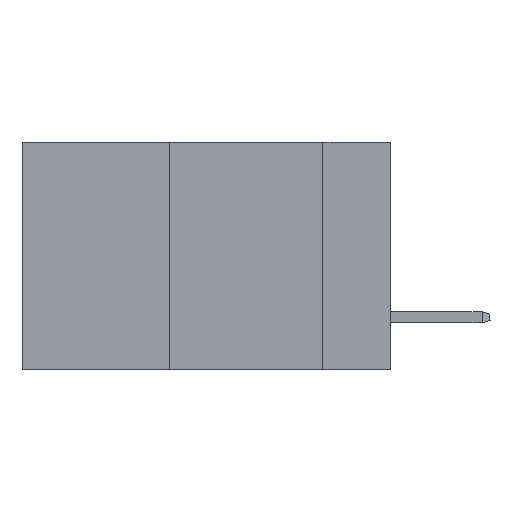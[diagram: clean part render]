
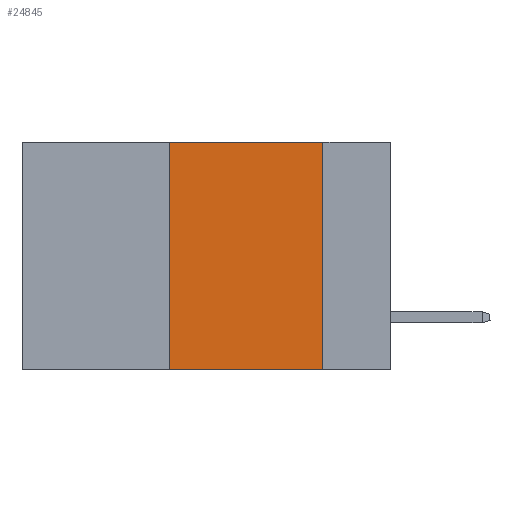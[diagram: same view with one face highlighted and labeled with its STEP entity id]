
A CAD part, left-side view. The second image highlights one B-rep face of the part: STEP entity #24845.
In plain terms, the highlighted planar face has unit normal (-1, 0, 0).
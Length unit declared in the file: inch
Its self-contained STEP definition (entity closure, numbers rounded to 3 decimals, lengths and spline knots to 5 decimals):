
#2 = LINE ( 'NONE', #37154, #11686 ) ;
#874 = DIRECTION ( 'NONE',  ( 0., 0., -1. ) ) ;
#4580 = EDGE_CURVE ( 'NONE', #42621, #16944, #2, .T. ) ;
#7854 = DIRECTION ( 'NONE',  ( 1., 0., 0. ) ) ;
#8788 = DIRECTION ( 'NONE',  ( 0., -1., 0. ) ) ;
#9383 = DIRECTION ( 'NONE',  ( 0., 0., -1. ) ) ;
#10991 = VECTOR ( 'NONE', #9383, 39.37008 ) ;
#11686 = VECTOR ( 'NONE', #8788, 39.37008 ) ;
#11754 = AXIS2_PLACEMENT_3D ( 'NONE', #18433, #7854, #874 ) ;
#13067 = CARTESIAN_POINT ( 'NONE',  ( 0., 0.36, 0. ) ) ;
#15099 = EDGE_CURVE ( 'NONE', #32289, #34947, #42749, .T. ) ;
#15758 = ORIENTED_EDGE ( 'NONE', *, *, #29307, .F. ) ;
#16707 = CARTESIAN_POINT ( 'NONE',  ( 0., 0.11, 0. ) ) ;
#16767 = EDGE_CURVE ( 'NONE', #34947, #16944, #44859, .T. ) ;
#16944 = VERTEX_POINT ( 'NONE', #39106 ) ;
#17495 = CARTESIAN_POINT ( 'NONE',  ( 0., 0.6, 0. ) ) ;
#18433 = CARTESIAN_POINT ( 'NONE',  ( 0., 0.6, 0. ) ) ;
#19946 = EDGE_LOOP ( 'NONE', ( #42183, #36063, #15758, #44729 ) ) ;
#22478 = CARTESIAN_POINT ( 'NONE',  ( 0., 0.36, -0.37 ) ) ;
#23125 = FACE_OUTER_BOUND ( 'NONE', #19946, .T. ) ;
#23761 = VECTOR ( 'NONE', #27941, 39.37008 ) ;
#24845 = ADVANCED_FACE ( 'NONE', ( #23125 ), #32059, .F. ) ;
#27941 = DIRECTION ( 'NONE',  ( 0., 0., 1. ) ) ;
#28200 = LINE ( 'NONE', #34598, #23761 ) ;
#29307 = EDGE_CURVE ( 'NONE', #42621, #32289, #28200, .T. ) ;
#32059 = PLANE ( 'NONE',  #11754 ) ;
#32289 = VERTEX_POINT ( 'NONE', #13067 ) ;
#33355 = VECTOR ( 'NONE', #35003, 39.37008 ) ;
#34598 = CARTESIAN_POINT ( 'NONE',  ( 0., 0.36, 0. ) ) ;
#34947 = VERTEX_POINT ( 'NONE', #39919 ) ;
#35003 = DIRECTION ( 'NONE',  ( 0., -1., 0. ) ) ;
#36063 = ORIENTED_EDGE ( 'NONE', *, *, #15099, .F. ) ;
#37154 = CARTESIAN_POINT ( 'NONE',  ( 0., 0.6, -0.37 ) ) ;
#39106 = CARTESIAN_POINT ( 'NONE',  ( 0., 0.11, -0.37 ) ) ;
#39919 = CARTESIAN_POINT ( 'NONE',  ( 0., 0.11, 0. ) ) ;
#42183 = ORIENTED_EDGE ( 'NONE', *, *, #16767, .F. ) ;
#42621 = VERTEX_POINT ( 'NONE', #22478 ) ;
#42749 = LINE ( 'NONE', #17495, #33355 ) ;
#44729 = ORIENTED_EDGE ( 'NONE', *, *, #4580, .T. ) ;
#44859 = LINE ( 'NONE', #16707, #10991 ) ;
